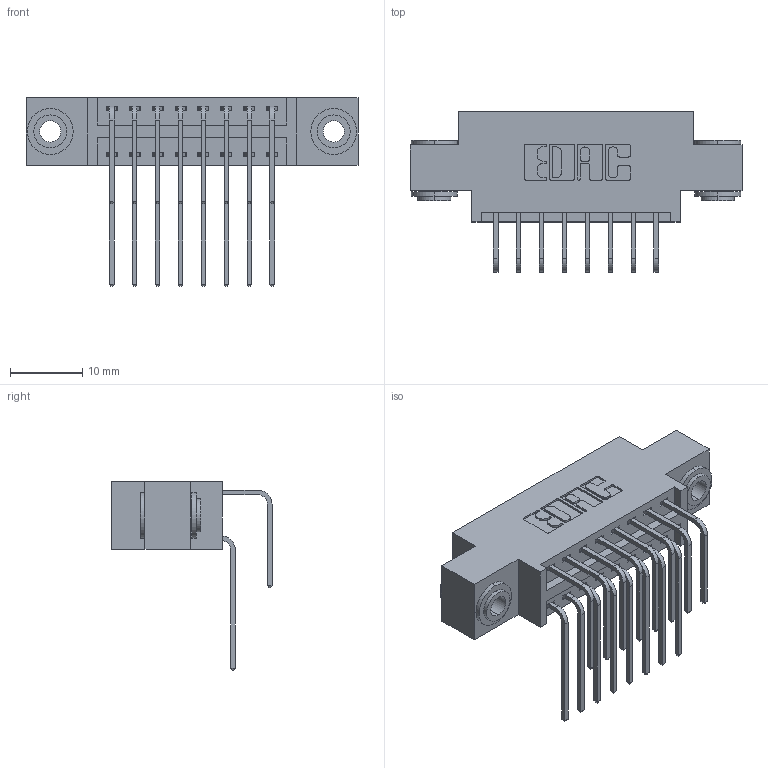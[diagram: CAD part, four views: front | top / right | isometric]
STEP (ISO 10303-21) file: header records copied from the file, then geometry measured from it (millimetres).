
FILE_DESCRIPTION (( 'STEP AP203' ), '1' );
FILE_NAME ('396-016-558-803.STEP', '2019-11-02T13:58:09', ( '' ), ( '' ), 'SwSTEP 2.0', 'SolidWorks 2016', '' );
FILE_SCHEMA (( 'CONFIG_CONTROL_DESIGN' ));
Length unit declared in the file: inch
Products named in the file (5): 345-250-002_345-250-002-102; 345-292-001_558 Tail - 2; 346 Part_0.170 Offset - 0.156 Dia-TH; 396-016-558-803; 345-292-001_558 559 Tail - 1
Assembly tree (19 placements, depth 2):
  396-016-558-803
    346 Part_0.170 Offset - 0.156 Dia-TH
    345-292-001_558 559 Tail - 1  x8
    345-292-001_558 Tail - 2  x8
    345-250-002_345-250-002-102  x2
Bounding box: 45.97 x 22.16 x 26.16 mm (x, y, z)
Volume: 4176 mm3; surface area: 6042.5 mm2
Topology: 19 solids, 19 shells, 1028 faces, 2993 edges, 1970 vertices
Faces by surface type: plane 682, cylinder 338, cone 8
Entity records: 12364 total; most frequent: CARTESIAN_POINT 2114, ORIENTED_EDGE 1990, DIRECTION 1917, EDGE_CURVE 995, VECTOR 767, LINE 767, VERTEX_POINT 658, AXIS2_PLACEMENT_3D 575
